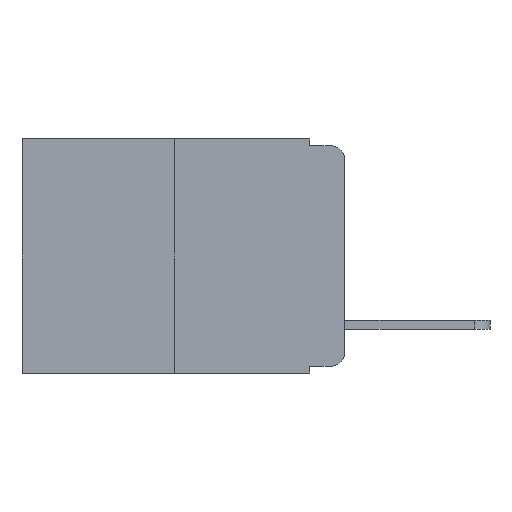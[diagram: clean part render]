
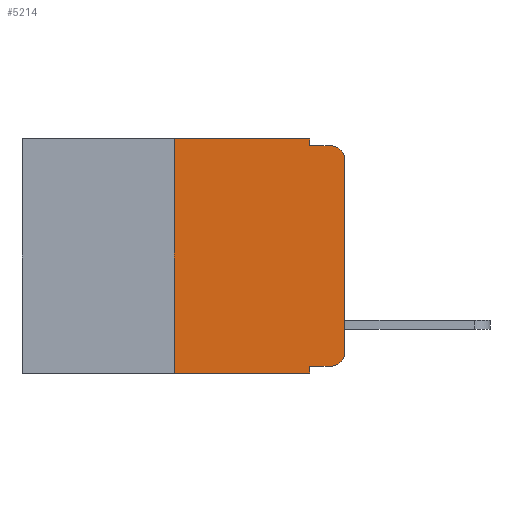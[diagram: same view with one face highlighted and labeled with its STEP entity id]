
A CAD part, left-side view. The second image highlights one B-rep face of the part: STEP entity #5214.
In plain terms, the highlighted planar face has unit normal (-1, 0, 0).
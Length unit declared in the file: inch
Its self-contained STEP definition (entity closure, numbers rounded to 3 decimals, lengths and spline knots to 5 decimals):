
#87 = ORIENTED_EDGE ( 'NONE', *, *, #21627, .F. ) ;
#153 = EDGE_CURVE ( 'NONE', #24613, #7614, #7300, .T. ) ;
#209 = EDGE_CURVE ( 'NONE', #6754, #25375, #11729, .T. ) ;
#442 = DIRECTION ( 'NONE',  ( 0., 0., -1. ) ) ;
#824 = EDGE_CURVE ( 'NONE', #21199, #25375, #5710, .T. ) ;
#1163 = CARTESIAN_POINT ( 'NONE',  ( 0., 0.051, -0.01 ) ) ;
#1306 = VECTOR ( 'NONE', #20899, 39.37008 ) ;
#1476 = CARTESIAN_POINT ( 'NONE',  ( 0., 0.25, 0. ) ) ;
#2452 = DIRECTION ( 'NONE',  ( -1., 0., 0. ) ) ;
#2874 = CARTESIAN_POINT ( 'NONE',  ( 0., 0., 0. ) ) ;
#3203 = AXIS2_PLACEMENT_3D ( 'NONE', #3247, #6382, #23187 ) ;
#3247 = CARTESIAN_POINT ( 'NONE',  ( 0., 0.473, 0. ) ) ;
#3722 = VERTEX_POINT ( 'NONE', #14757 ) ;
#3875 = EDGE_CURVE ( 'NONE', #7614, #8383, #4101, .T. ) ;
#4101 = LINE ( 'NONE', #1163, #15472 ) ;
#4749 = CARTESIAN_POINT ( 'NONE',  ( 0., 0.25, 0. ) ) ;
#5057 = DIRECTION ( 'NONE',  ( -1., 0., 0. ) ) ;
#5062 = DIRECTION ( 'NONE',  ( 0., -1., 0. ) ) ;
#5214 = ADVANCED_FACE ( 'NONE', ( #13508 ), #7979, .F. ) ;
#5253 = VERTEX_POINT ( 'NONE', #15366 ) ;
#5593 = DIRECTION ( 'NONE',  ( 0., -1., 0. ) ) ;
#5607 = EDGE_CURVE ( 'NONE', #3722, #5253, #15059, .T. ) ;
#5710 = LINE ( 'NONE', #12386, #18629 ) ;
#5902 = LINE ( 'NONE', #15815, #19153 ) ;
#6077 = ORIENTED_EDGE ( 'NONE', *, *, #19289, .T. ) ;
#6183 = LINE ( 'NONE', #1476, #8056 ) ;
#6208 = CARTESIAN_POINT ( 'NONE',  ( 0., 0., -0.03 ) ) ;
#6382 = DIRECTION ( 'NONE',  ( 1., 0., 0. ) ) ;
#6492 = CARTESIAN_POINT ( 'NONE',  ( 0., 0.051, -0.01 ) ) ;
#6658 = CARTESIAN_POINT ( 'NONE',  ( 0., 0.25, -0.343 ) ) ;
#6697 = CARTESIAN_POINT ( 'NONE',  ( 0., 0.051, -0.343 ) ) ;
#6754 = VERTEX_POINT ( 'NONE', #6658 ) ;
#7300 = LINE ( 'NONE', #22745, #1306 ) ;
#7374 = DIRECTION ( 'NONE',  ( 0., 0., 1. ) ) ;
#7614 = VERTEX_POINT ( 'NONE', #6492 ) ;
#7979 = PLANE ( 'NONE',  #3203 ) ;
#8056 = VECTOR ( 'NONE', #7374, 39.37008 ) ;
#8383 = VERTEX_POINT ( 'NONE', #19470 ) ;
#8508 = DIRECTION ( 'NONE',  ( 0., -1., 0. ) ) ;
#8833 = ORIENTED_EDGE ( 'NONE', *, *, #153, .F. ) ;
#8893 = CARTESIAN_POINT ( 'NONE',  ( 0., 0.02, -0.313 ) ) ;
#9090 = DIRECTION ( 'NONE',  ( 0., 0., -1. ) ) ;
#9756 = VERTEX_POINT ( 'NONE', #4749 ) ;
#9974 = EDGE_CURVE ( 'NONE', #6754, #9756, #6183, .T. ) ;
#10481 = CARTESIAN_POINT ( 'NONE',  ( 0., 0.02, -0.03 ) ) ;
#10830 = ORIENTED_EDGE ( 'NONE', *, *, #824, .F. ) ;
#11389 = AXIS2_PLACEMENT_3D ( 'NONE', #10481, #2452, #16577 ) ;
#11417 = VECTOR ( 'NONE', #8508, 39.37008 ) ;
#11729 = LINE ( 'NONE', #12254, #11417 ) ;
#12028 = AXIS2_PLACEMENT_3D ( 'NONE', #8893, #5057, #9090 ) ;
#12254 = CARTESIAN_POINT ( 'NONE',  ( 0., 0.473, -0.343 ) ) ;
#12373 = CARTESIAN_POINT ( 'NONE',  ( 0., 0.051, -0.333 ) ) ;
#12386 = CARTESIAN_POINT ( 'NONE',  ( 0., 0.051, 0. ) ) ;
#13150 = DIRECTION ( 'NONE',  ( 0., -1., 0. ) ) ;
#13508 = FACE_OUTER_BOUND ( 'NONE', #16113, .T. ) ;
#13571 = ORIENTED_EDGE ( 'NONE', *, *, #19603, .T. ) ;
#14757 = CARTESIAN_POINT ( 'NONE',  ( 0., 0.02, -0.333 ) ) ;
#14995 = ORIENTED_EDGE ( 'NONE', *, *, #17839, .T. ) ;
#15059 = CIRCLE ( 'NONE', #12028, 0.02 ) ;
#15252 = DIRECTION ( 'NONE',  ( 0., 0., 1. ) ) ;
#15366 = CARTESIAN_POINT ( 'NONE',  ( 0., 0., -0.313 ) ) ;
#15429 = VECTOR ( 'NONE', #13150, 39.37008 ) ;
#15472 = VECTOR ( 'NONE', #5062, 39.37008 ) ;
#15815 = CARTESIAN_POINT ( 'NONE',  ( 0., 0.473, 0. ) ) ;
#15842 = ORIENTED_EDGE ( 'NONE', *, *, #9974, .F. ) ;
#15881 = ORIENTED_EDGE ( 'NONE', *, *, #209, .T. ) ;
#16113 = EDGE_LOOP ( 'NONE', ( #6077, #13571, #20344, #8833, #87, #15842, #15881, #10830, #14995, #21392 ) ) ;
#16577 = DIRECTION ( 'NONE',  ( 0., 0., -1. ) ) ;
#17288 = VECTOR ( 'NONE', #15252, 39.37008 ) ;
#17624 = LINE ( 'NONE', #2874, #17288 ) ;
#17839 = EDGE_CURVE ( 'NONE', #21199, #3722, #22676, .T. ) ;
#18629 = VECTOR ( 'NONE', #442, 39.37008 ) ;
#18969 = CARTESIAN_POINT ( 'NONE',  ( 0., 0.051, -0.333 ) ) ;
#19153 = VECTOR ( 'NONE', #5593, 39.37008 ) ;
#19289 = EDGE_CURVE ( 'NONE', #5253, #23715, #17624, .T. ) ;
#19470 = CARTESIAN_POINT ( 'NONE',  ( 0., 0.02, -0.01 ) ) ;
#19603 = EDGE_CURVE ( 'NONE', #23715, #8383, #24205, .T. ) ;
#20344 = ORIENTED_EDGE ( 'NONE', *, *, #3875, .F. ) ;
#20899 = DIRECTION ( 'NONE',  ( 0., 0., -1. ) ) ;
#21199 = VERTEX_POINT ( 'NONE', #12373 ) ;
#21373 = CARTESIAN_POINT ( 'NONE',  ( 0., 0.051, 0. ) ) ;
#21392 = ORIENTED_EDGE ( 'NONE', *, *, #5607, .T. ) ;
#21627 = EDGE_CURVE ( 'NONE', #9756, #24613, #5902, .T. ) ;
#22676 = LINE ( 'NONE', #18969, #15429 ) ;
#22745 = CARTESIAN_POINT ( 'NONE',  ( 0., 0.051, 0. ) ) ;
#23187 = DIRECTION ( 'NONE',  ( 0., 0., -1. ) ) ;
#23715 = VERTEX_POINT ( 'NONE', #6208 ) ;
#24205 = CIRCLE ( 'NONE', #11389, 0.02 ) ;
#24613 = VERTEX_POINT ( 'NONE', #21373 ) ;
#25375 = VERTEX_POINT ( 'NONE', #6697 ) ;
